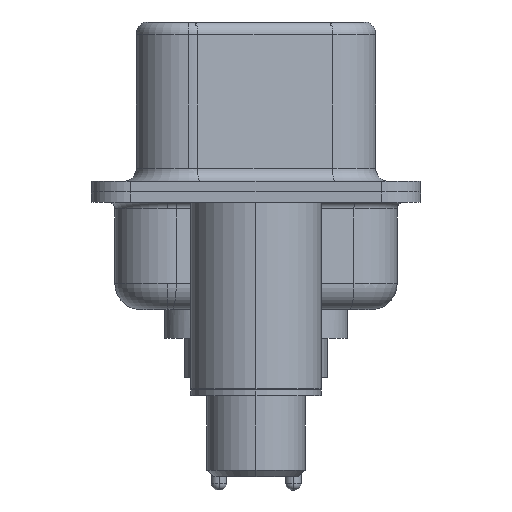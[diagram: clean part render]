
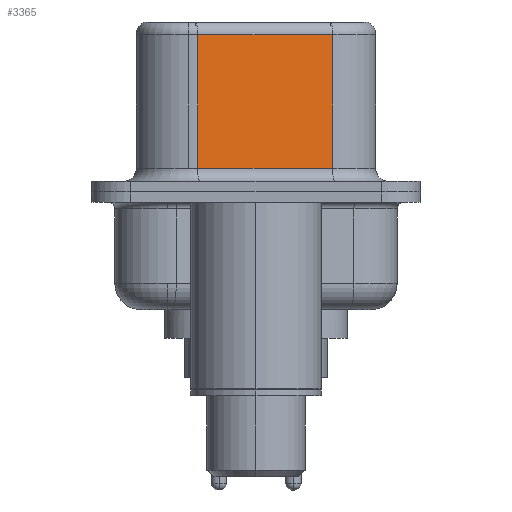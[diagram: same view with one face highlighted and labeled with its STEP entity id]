
A CAD part, left-side view. The second image highlights one B-rep face of the part: STEP entity #3365.
In plain terms, the highlighted planar face has unit normal (-0.985, -0.174, 0).
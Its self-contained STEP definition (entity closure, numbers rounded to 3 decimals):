
#370 = ORIENTED_EDGE ( 'NONE', *, *, #8997, .T. ) ;
#541 = CARTESIAN_POINT ( 'NONE',  ( 4.58, -2.927, 0.9 ) ) ;
#2113 = VECTOR ( 'NONE', #7588, 1000. ) ;
#2207 = CARTESIAN_POINT ( 'NONE',  ( 4.58, -2.927, 6.52 ) ) ;
#3269 = LINE ( 'NONE', #24605, #24761 ) ;
#3365 = ADVANCED_FACE ( 'NONE', ( #18696 ), #22093, .F. ) ;
#3974 = DIRECTION ( 'NONE',  ( 0.985, 0.174, 0. ) ) ;
#4981 = ORIENTED_EDGE ( 'NONE', *, *, #6184, .T. ) ;
#5056 = VERTEX_POINT ( 'NONE', #541 ) ;
#5268 = LINE ( 'NONE', #21453, #26667 ) ;
#5418 = CARTESIAN_POINT ( 'NONE',  ( 4.58, -2.927, 6.02 ) ) ;
#5560 = EDGE_LOOP ( 'NONE', ( #15204, #370, #6482, #4981 ) ) ;
#5986 = DIRECTION ( 'NONE',  ( 0., 0., -1. ) ) ;
#6184 = EDGE_CURVE ( 'NONE', #7445, #5056, #21878, .T. ) ;
#6255 = VERTEX_POINT ( 'NONE', #10037 ) ;
#6482 = ORIENTED_EDGE ( 'NONE', *, *, #18066, .T. ) ;
#7290 = AXIS2_PLACEMENT_3D ( 'NONE', #2207, #3974, #14966 ) ;
#7445 = VERTEX_POINT ( 'NONE', #7620 ) ;
#7588 = DIRECTION ( 'NONE',  ( -0.174, 0.985, 0. ) ) ;
#7620 = CARTESIAN_POINT ( 'NONE',  ( 3.67, 2.233, 0.9 ) ) ;
#8997 = EDGE_CURVE ( 'NONE', #6255, #24747, #13385, .T. ) ;
#10037 = CARTESIAN_POINT ( 'NONE',  ( 4.58, -2.927, 6.02 ) ) ;
#13385 = LINE ( 'NONE', #5418, #2113 ) ;
#14966 = DIRECTION ( 'NONE',  ( -0.174, 0.985, 0. ) ) ;
#15204 = ORIENTED_EDGE ( 'NONE', *, *, #18868, .F. ) ;
#15387 = DIRECTION ( 'NONE',  ( 0., 0., -1. ) ) ;
#16464 = VECTOR ( 'NONE', #26253, 1000. ) ;
#18066 = EDGE_CURVE ( 'NONE', #24747, #7445, #3269, .T. ) ;
#18696 = FACE_OUTER_BOUND ( 'NONE', #5560, .T. ) ;
#18868 = EDGE_CURVE ( 'NONE', #6255, #5056, #5268, .T. ) ;
#20097 = CARTESIAN_POINT ( 'NONE',  ( 3.67, 2.233, 6.02 ) ) ;
#20190 = CARTESIAN_POINT ( 'NONE',  ( 4.58, -2.927, 0.9 ) ) ;
#21453 = CARTESIAN_POINT ( 'NONE',  ( 4.58, -2.927, 6.52 ) ) ;
#21878 = LINE ( 'NONE', #20190, #16464 ) ;
#22093 = PLANE ( 'NONE',  #7290 ) ;
#24605 = CARTESIAN_POINT ( 'NONE',  ( 3.67, 2.233, 6.52 ) ) ;
#24747 = VERTEX_POINT ( 'NONE', #20097 ) ;
#24761 = VECTOR ( 'NONE', #5986, 1000. ) ;
#26253 = DIRECTION ( 'NONE',  ( 0.174, -0.985, 0. ) ) ;
#26667 = VECTOR ( 'NONE', #15387, 1000. ) ;
